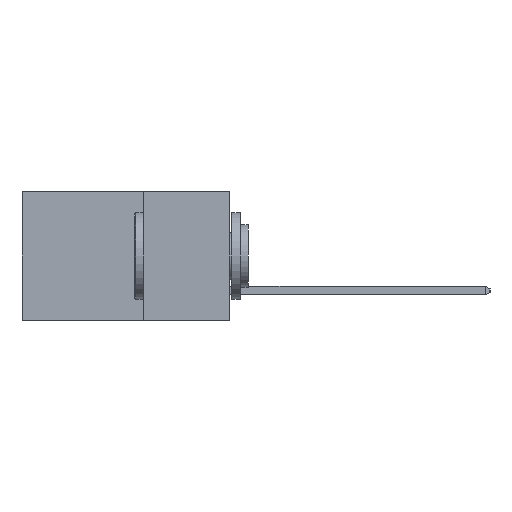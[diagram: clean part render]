
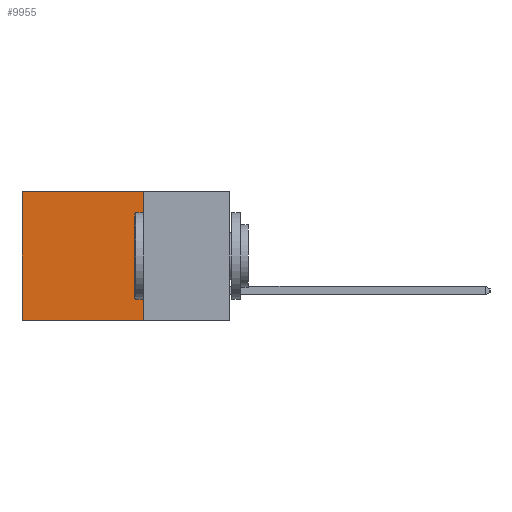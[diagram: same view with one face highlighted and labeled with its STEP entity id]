
A CAD part, left-side view. The second image highlights one B-rep face of the part: STEP entity #9955.
In plain terms, the highlighted planar face has unit normal (-1, 0, 0).
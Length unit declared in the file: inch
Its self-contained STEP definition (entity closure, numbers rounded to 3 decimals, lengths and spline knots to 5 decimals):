
#62 = DIRECTION ( 'NONE',  ( 1., 0., 0. ) ) ;
#883 = CARTESIAN_POINT ( 'NONE',  ( 0.298, 0.25, -0.37 ) ) ;
#1507 = LINE ( 'NONE', #6863, #12675 ) ;
#2208 = EDGE_CURVE ( 'NONE', #8744, #12158, #4369, .T. ) ;
#2281 = DIRECTION ( 'NONE',  ( 0., 0., -1. ) ) ;
#2591 = DIRECTION ( 'NONE',  ( 0., 0., -1. ) ) ;
#2629 = CARTESIAN_POINT ( 'NONE',  ( 0.298, 0.6, 0. ) ) ;
#3142 = CARTESIAN_POINT ( 'NONE',  ( 0.298, 0.25, -0.37 ) ) ;
#3436 = CARTESIAN_POINT ( 'NONE',  ( 0.298, 0.25, 0. ) ) ;
#4369 = LINE ( 'NONE', #2629, #12243 ) ;
#4617 = PLANE ( 'NONE',  #6776 ) ;
#4759 = LINE ( 'NONE', #883, #7428 ) ;
#4863 = VERTEX_POINT ( 'NONE', #3142 ) ;
#5353 = EDGE_CURVE ( 'NONE', #4863, #12158, #4759, .T. ) ;
#6776 = AXIS2_PLACEMENT_3D ( 'NONE', #3436, #62, #8013 ) ;
#6863 = CARTESIAN_POINT ( 'NONE',  ( 0.298, 0.25, 0. ) ) ;
#7015 = VERTEX_POINT ( 'NONE', #7297 ) ;
#7059 = ORIENTED_EDGE ( 'NONE', *, *, #2208, .T. ) ;
#7297 = CARTESIAN_POINT ( 'NONE',  ( 0.298, 0.25, 0. ) ) ;
#7428 = VECTOR ( 'NONE', #13203, 39.37008 ) ;
#8013 = DIRECTION ( 'NONE',  ( 0., 0., -1. ) ) ;
#8286 = ORIENTED_EDGE ( 'NONE', *, *, #5353, .F. ) ;
#8432 = CARTESIAN_POINT ( 'NONE',  ( 0.298, 0.25, 0. ) ) ;
#8744 = VERTEX_POINT ( 'NONE', #10155 ) ;
#8953 = ORIENTED_EDGE ( 'NONE', *, *, #12101, .F. ) ;
#9480 = FACE_OUTER_BOUND ( 'NONE', #12264, .T. ) ;
#9955 = ADVANCED_FACE ( 'NONE', ( #9480 ), #4617, .F. ) ;
#10155 = CARTESIAN_POINT ( 'NONE',  ( 0.298, 0.6, 0. ) ) ;
#10222 = CARTESIAN_POINT ( 'NONE',  ( 0.298, 0.6, -0.37 ) ) ;
#10653 = ORIENTED_EDGE ( 'NONE', *, *, #10855, .T. ) ;
#10855 = EDGE_CURVE ( 'NONE', #7015, #8744, #13708, .T. ) ;
#12101 = EDGE_CURVE ( 'NONE', #7015, #4863, #1507, .T. ) ;
#12158 = VERTEX_POINT ( 'NONE', #10222 ) ;
#12243 = VECTOR ( 'NONE', #2591, 39.37008 ) ;
#12264 = EDGE_LOOP ( 'NONE', ( #7059, #8286, #8953, #10653 ) ) ;
#12675 = VECTOR ( 'NONE', #2281, 39.37008 ) ;
#13203 = DIRECTION ( 'NONE',  ( 0., 1., 0. ) ) ;
#13387 = DIRECTION ( 'NONE',  ( 0., 1., 0. ) ) ;
#13409 = VECTOR ( 'NONE', #13387, 39.37008 ) ;
#13708 = LINE ( 'NONE', #8432, #13409 ) ;
